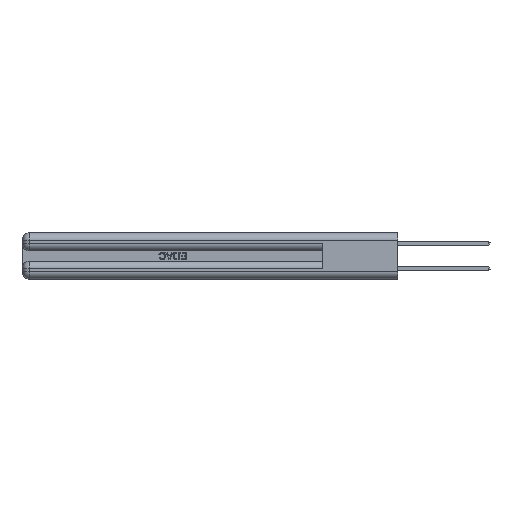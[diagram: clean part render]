
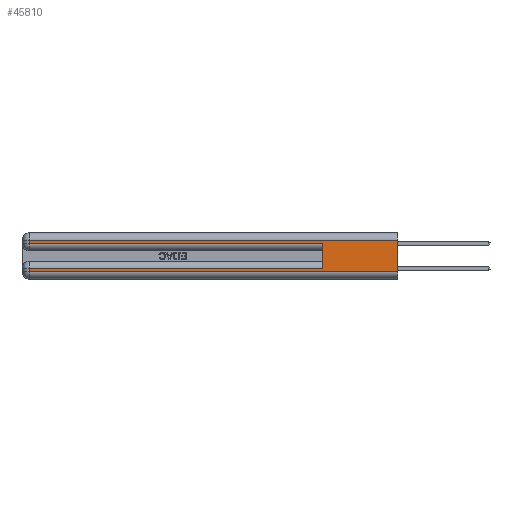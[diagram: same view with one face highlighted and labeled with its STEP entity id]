
A CAD part, left-side view. The second image highlights one B-rep face of the part: STEP entity #45810.
In plain terms, the highlighted planar face has unit normal (-1, 0, 0).
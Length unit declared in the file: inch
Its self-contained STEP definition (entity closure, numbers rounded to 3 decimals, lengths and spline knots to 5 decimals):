
#450 = VERTEX_POINT ( 'NONE', #32488 ) ;
#722 = FACE_OUTER_BOUND ( 'NONE', #31504, .T. ) ;
#1097 = LINE ( 'NONE', #38154, #10045 ) ;
#1253 = VECTOR ( 'NONE', #28977, 39.37008 ) ;
#1386 = LINE ( 'NONE', #35341, #40529 ) ;
#1938 = CARTESIAN_POINT ( 'NONE',  ( 0., 0., 0.06 ) ) ;
#3894 = EDGE_CURVE ( 'NONE', #39348, #46631, #38345, .T. ) ;
#6008 = ORIENTED_EDGE ( 'NONE', *, *, #36963, .T. ) ;
#7690 = CARTESIAN_POINT ( 'NONE',  ( 0., 0., 0.31 ) ) ;
#8024 = EDGE_CURVE ( 'NONE', #28335, #21703, #28082, .T. ) ;
#9342 = CARTESIAN_POINT ( 'NONE',  ( 0., 0., 0.31 ) ) ;
#10045 = VECTOR ( 'NONE', #45701, 39.37008 ) ;
#10069 = CARTESIAN_POINT ( 'NONE',  ( 0., 0., 0.06 ) ) ;
#10162 = CARTESIAN_POINT ( 'NONE',  ( 0., 2.94, 0.285 ) ) ;
#10967 = CARTESIAN_POINT ( 'NONE',  ( 0., 2.94, 0.06 ) ) ;
#11342 = ORIENTED_EDGE ( 'NONE', *, *, #20787, .F. ) ;
#12205 = EDGE_CURVE ( 'NONE', #43718, #39152, #36598, .T. ) ;
#12645 = DIRECTION ( 'NONE',  ( 0., 0., 1. ) ) ;
#13360 = CARTESIAN_POINT ( 'NONE',  ( 0., 0., 0.37 ) ) ;
#14000 = DIRECTION ( 'NONE',  ( 0., -1., 0. ) ) ;
#16835 = VECTOR ( 'NONE', #14000, 39.37008 ) ;
#17840 = DIRECTION ( 'NONE',  ( 0., 0., -1. ) ) ;
#17877 = ORIENTED_EDGE ( 'NONE', *, *, #41062, .T. ) ;
#20213 = ORIENTED_EDGE ( 'NONE', *, *, #12205, .F. ) ;
#20787 = EDGE_CURVE ( 'NONE', #450, #21703, #1386, .T. ) ;
#21169 = VECTOR ( 'NONE', #32319, 39.37008 ) ;
#21478 = LINE ( 'NONE', #25154, #1253 ) ;
#21703 = VERTEX_POINT ( 'NONE', #36903 ) ;
#22486 = CARTESIAN_POINT ( 'NONE',  ( 0., 2.94, 0.085 ) ) ;
#23523 = LINE ( 'NONE', #1938, #21169 ) ;
#24230 = EDGE_CURVE ( 'NONE', #450, #39348, #1097, .T. ) ;
#25154 = CARTESIAN_POINT ( 'NONE',  ( 0., 2.94, 0.37 ) ) ;
#25854 = EDGE_CURVE ( 'NONE', #43718, #41480, #43041, .T. ) ;
#28082 = LINE ( 'NONE', #44090, #16835 ) ;
#28335 = VERTEX_POINT ( 'NONE', #10162 ) ;
#28421 = DIRECTION ( 'NONE',  ( 0., 1., 0. ) ) ;
#28977 = DIRECTION ( 'NONE',  ( 0., 0., -1. ) ) ;
#30288 = ORIENTED_EDGE ( 'NONE', *, *, #25854, .T. ) ;
#30650 = VECTOR ( 'NONE', #28421, 39.37008 ) ;
#31504 = EDGE_LOOP ( 'NONE', ( #20213, #30288, #17877, #40364, #11342, #31527, #35065, #6008 ) ) ;
#31527 = ORIENTED_EDGE ( 'NONE', *, *, #24230, .T. ) ;
#32227 = CARTESIAN_POINT ( 'NONE',  ( 0., 2.94, 0.37 ) ) ;
#32319 = DIRECTION ( 'NONE',  ( 0., -1., 0. ) ) ;
#32488 = CARTESIAN_POINT ( 'NONE',  ( 0., 0.6, 0.085 ) ) ;
#32917 = PLANE ( 'NONE',  #45930 ) ;
#35059 = CARTESIAN_POINT ( 'NONE',  ( 0., 2.94, 0.31 ) ) ;
#35065 = ORIENTED_EDGE ( 'NONE', *, *, #3894, .T. ) ;
#35341 = CARTESIAN_POINT ( 'NONE',  ( 0., 0.6, 0.145 ) ) ;
#35410 = VECTOR ( 'NONE', #47297, 39.37008 ) ;
#36004 = DIRECTION ( 'NONE',  ( 0., 0., -1. ) ) ;
#36598 = LINE ( 'NONE', #43556, #35410 ) ;
#36903 = CARTESIAN_POINT ( 'NONE',  ( 0., 0.6, 0.285 ) ) ;
#36963 = EDGE_CURVE ( 'NONE', #46631, #39152, #23523, .T. ) ;
#38154 = CARTESIAN_POINT ( 'NONE',  ( 0., 0., 0.085 ) ) ;
#38345 = LINE ( 'NONE', #32227, #45966 ) ;
#39152 = VERTEX_POINT ( 'NONE', #10069 ) ;
#39348 = VERTEX_POINT ( 'NONE', #22486 ) ;
#40364 = ORIENTED_EDGE ( 'NONE', *, *, #8024, .T. ) ;
#40501 = DIRECTION ( 'NONE',  ( 1., 0., 0. ) ) ;
#40529 = VECTOR ( 'NONE', #12645, 39.37008 ) ;
#41062 = EDGE_CURVE ( 'NONE', #41480, #28335, #21478, .T. ) ;
#41480 = VERTEX_POINT ( 'NONE', #35059 ) ;
#43041 = LINE ( 'NONE', #9342, #30650 ) ;
#43556 = CARTESIAN_POINT ( 'NONE',  ( 0., 0., 0.37 ) ) ;
#43718 = VERTEX_POINT ( 'NONE', #7690 ) ;
#44090 = CARTESIAN_POINT ( 'NONE',  ( 0., 0., 0.285 ) ) ;
#45701 = DIRECTION ( 'NONE',  ( 0., 1., 0. ) ) ;
#45810 = ADVANCED_FACE ( 'NONE', ( #722 ), #32917, .F. ) ;
#45930 = AXIS2_PLACEMENT_3D ( 'NONE', #13360, #40501, #17840 ) ;
#45966 = VECTOR ( 'NONE', #36004, 39.37008 ) ;
#46631 = VERTEX_POINT ( 'NONE', #10967 ) ;
#47297 = DIRECTION ( 'NONE',  ( 0., 0., -1. ) ) ;
